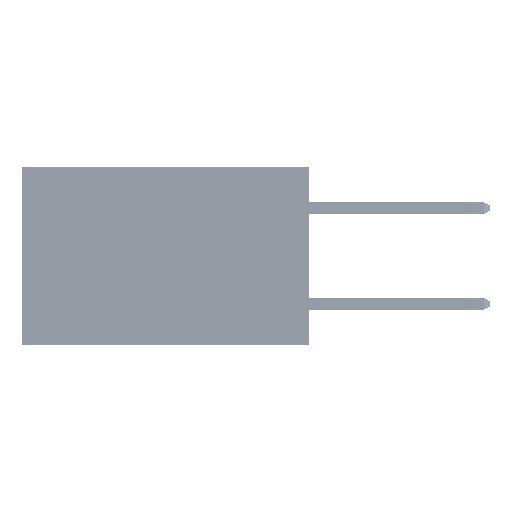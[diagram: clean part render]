
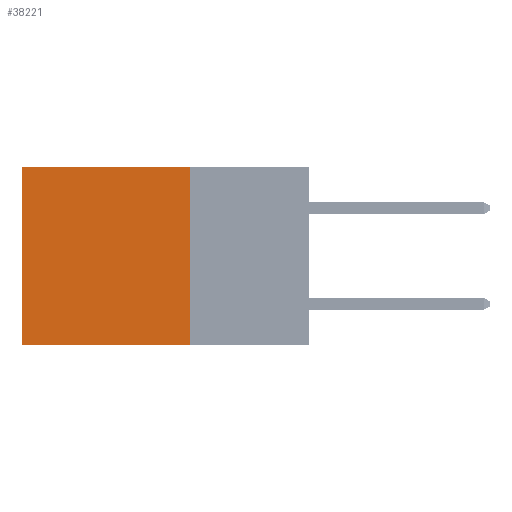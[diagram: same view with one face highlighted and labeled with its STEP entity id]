
A CAD part, left-side view. The second image highlights one B-rep face of the part: STEP entity #38221.
In plain terms, the highlighted planar face has unit normal (-1, 0, 0).
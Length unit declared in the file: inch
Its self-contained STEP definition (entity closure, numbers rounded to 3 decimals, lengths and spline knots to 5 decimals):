
#2757 = VECTOR ( 'NONE', #41812, 39.37008 ) ;
#3044 = FACE_OUTER_BOUND ( 'NONE', #26672, .T. ) ;
#4014 = CARTESIAN_POINT ( 'NONE',  ( 0.2875, 0.25, -0.37 ) ) ;
#6440 = VERTEX_POINT ( 'NONE', #13282 ) ;
#8062 = CARTESIAN_POINT ( 'NONE',  ( 0.2875, 0.6, -0.37 ) ) ;
#8552 = ORIENTED_EDGE ( 'NONE', *, *, #38927, .T. ) ;
#10929 = PLANE ( 'NONE',  #13002 ) ;
#13002 = AXIS2_PLACEMENT_3D ( 'NONE', #26220, #45345, #45602 ) ;
#13282 = CARTESIAN_POINT ( 'NONE',  ( 0.2875, 0.25, 0. ) ) ;
#13400 = VERTEX_POINT ( 'NONE', #4014 ) ;
#14549 = CARTESIAN_POINT ( 'NONE',  ( 0.2875, 0.25, -0.37 ) ) ;
#15815 = CARTESIAN_POINT ( 'NONE',  ( 0.2875, 0.6, 0. ) ) ;
#16051 = ORIENTED_EDGE ( 'NONE', *, *, #41749, .T. ) ;
#20897 = EDGE_CURVE ( 'NONE', #6440, #13400, #22915, .T. ) ;
#22865 = VERTEX_POINT ( 'NONE', #8062 ) ;
#22915 = LINE ( 'NONE', #49951, #35484 ) ;
#23231 = LINE ( 'NONE', #14549, #25366 ) ;
#25366 = VECTOR ( 'NONE', #38777, 39.37008 ) ;
#26220 = CARTESIAN_POINT ( 'NONE',  ( 0.2875, 0.25, 0. ) ) ;
#26257 = CARTESIAN_POINT ( 'NONE',  ( 0.2875, 0.25, 0. ) ) ;
#26672 = EDGE_LOOP ( 'NONE', ( #8552, #47315, #40842, #16051 ) ) ;
#30059 = DIRECTION ( 'NONE',  ( 0., 0., -1. ) ) ;
#30082 = LINE ( 'NONE', #26257, #2757 ) ;
#31034 = VERTEX_POINT ( 'NONE', #15815 ) ;
#31241 = CARTESIAN_POINT ( 'NONE',  ( 0.2875, 0.6, 0. ) ) ;
#35064 = LINE ( 'NONE', #31241, #49733 ) ;
#35484 = VECTOR ( 'NONE', #30059, 39.37008 ) ;
#38221 = ADVANCED_FACE ( 'NONE', ( #3044 ), #10929, .F. ) ;
#38777 = DIRECTION ( 'NONE',  ( 0., 1., 0. ) ) ;
#38927 = EDGE_CURVE ( 'NONE', #31034, #22865, #35064, .T. ) ;
#39798 = EDGE_CURVE ( 'NONE', #13400, #22865, #23231, .T. ) ;
#40842 = ORIENTED_EDGE ( 'NONE', *, *, #20897, .F. ) ;
#41749 = EDGE_CURVE ( 'NONE', #6440, #31034, #30082, .T. ) ;
#41812 = DIRECTION ( 'NONE',  ( 0., 1., 0. ) ) ;
#45345 = DIRECTION ( 'NONE',  ( 1., 0., 0. ) ) ;
#45602 = DIRECTION ( 'NONE',  ( 0., 0., -1. ) ) ;
#46780 = DIRECTION ( 'NONE',  ( 0., 0., -1. ) ) ;
#47315 = ORIENTED_EDGE ( 'NONE', *, *, #39798, .F. ) ;
#49733 = VECTOR ( 'NONE', #46780, 39.37008 ) ;
#49951 = CARTESIAN_POINT ( 'NONE',  ( 0.2875, 0.25, 0. ) ) ;
